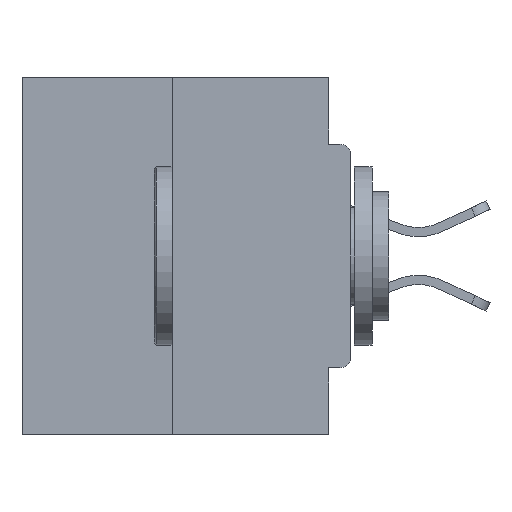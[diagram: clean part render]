
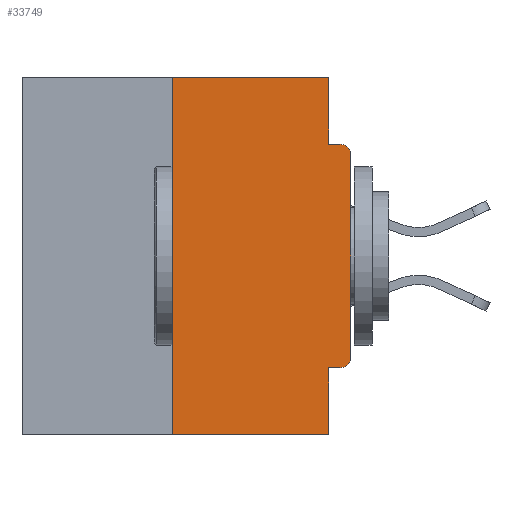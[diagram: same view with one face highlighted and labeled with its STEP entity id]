
A CAD part, left-side view. The second image highlights one B-rep face of the part: STEP entity #33749.
In plain terms, the highlighted planar face has unit normal (-1, 0, 0).
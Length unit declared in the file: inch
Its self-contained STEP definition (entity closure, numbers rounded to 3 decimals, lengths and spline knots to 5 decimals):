
#339 = DIRECTION ( 'NONE',  ( 0., 0., -1. ) ) ;
#529 = VERTEX_POINT ( 'NONE', #2302 ) ;
#733 = DIRECTION ( 'NONE',  ( 0., 0., -1. ) ) ;
#1420 = VECTOR ( 'NONE', #32001, 39.37008 ) ;
#1704 = CIRCLE ( 'NONE', #24526, 0.015 ) ;
#2302 = CARTESIAN_POINT ( 'NONE',  ( 0., 0.031, -0.5 ) ) ;
#2428 = VERTEX_POINT ( 'NONE', #33903 ) ;
#2849 = ORIENTED_EDGE ( 'NONE', *, *, #25005, .F. ) ;
#3294 = EDGE_CURVE ( 'NONE', #30026, #2428, #1704, .T. ) ;
#3412 = CARTESIAN_POINT ( 'NONE',  ( 0., 0.015, -0.3915 ) ) ;
#3542 = PLANE ( 'NONE',  #29094 ) ;
#4584 = ORIENTED_EDGE ( 'NONE', *, *, #19382, .F. ) ;
#4960 = CARTESIAN_POINT ( 'NONE',  ( 0., 0.46, 0. ) ) ;
#5961 = CARTESIAN_POINT ( 'NONE',  ( 0., 0., -0.0935 ) ) ;
#6824 = CARTESIAN_POINT ( 'NONE',  ( 0., 0.015, -0.1085 ) ) ;
#7089 = VECTOR ( 'NONE', #10782, 39.37008 ) ;
#8106 = LINE ( 'NONE', #30395, #28964 ) ;
#8495 = CARTESIAN_POINT ( 'NONE',  ( 0., 0.015, -0.4065 ) ) ;
#8805 = DIRECTION ( 'NONE',  ( 0., -1., 0. ) ) ;
#8964 = ORIENTED_EDGE ( 'NONE', *, *, #31930, .F. ) ;
#10055 = VECTOR ( 'NONE', #21540, 39.37008 ) ;
#10618 = CARTESIAN_POINT ( 'NONE',  ( 0., 0.25, 0. ) ) ;
#10782 = DIRECTION ( 'NONE',  ( 0., -1., 0. ) ) ;
#11637 = CIRCLE ( 'NONE', #35194, 0.015 ) ;
#11740 = ORIENTED_EDGE ( 'NONE', *, *, #20751, .T. ) ;
#13458 = VERTEX_POINT ( 'NONE', #14310 ) ;
#13988 = CARTESIAN_POINT ( 'NONE',  ( 0., 0.46, 0. ) ) ;
#14027 = DIRECTION ( 'NONE',  ( 0., 0., 1. ) ) ;
#14169 = DIRECTION ( 'NONE',  ( 0., 1., 0. ) ) ;
#14310 = CARTESIAN_POINT ( 'NONE',  ( 0., 0.031, -0.4065 ) ) ;
#15445 = CARTESIAN_POINT ( 'NONE',  ( 0., 0.015, -0.0935 ) ) ;
#15452 = CARTESIAN_POINT ( 'NONE',  ( 0., 0.031, 0. ) ) ;
#16321 = ORIENTED_EDGE ( 'NONE', *, *, #34888, .T. ) ;
#16607 = DIRECTION ( 'NONE',  ( 0., 0., -1. ) ) ;
#16608 = FACE_OUTER_BOUND ( 'NONE', #26049, .T. ) ;
#16656 = VECTOR ( 'NONE', #14169, 39.37008 ) ;
#17760 = EDGE_CURVE ( 'NONE', #19184, #34465, #28795, .T. ) ;
#18107 = DIRECTION ( 'NONE',  ( 0., 0., -1. ) ) ;
#18458 = EDGE_CURVE ( 'NONE', #34465, #23523, #22446, .T. ) ;
#18556 = LINE ( 'NONE', #5961, #33885 ) ;
#18764 = LINE ( 'NONE', #19774, #16656 ) ;
#19184 = VERTEX_POINT ( 'NONE', #27040 ) ;
#19209 = EDGE_CURVE ( 'NONE', #23523, #33570, #18556, .T. ) ;
#19382 = EDGE_CURVE ( 'NONE', #28916, #19184, #31724, .T. ) ;
#19695 = DIRECTION ( 'NONE',  ( -1., 0., 0. ) ) ;
#19774 = CARTESIAN_POINT ( 'NONE',  ( 0., 0., -0.4065 ) ) ;
#19952 = CARTESIAN_POINT ( 'NONE',  ( 0., 0.031, 0. ) ) ;
#20751 = EDGE_CURVE ( 'NONE', #25872, #33570, #11637, .T. ) ;
#21434 = CARTESIAN_POINT ( 'NONE',  ( 0., 0.25, -0.5 ) ) ;
#21540 = DIRECTION ( 'NONE',  ( 0., 0., 1. ) ) ;
#21894 = EDGE_CURVE ( 'NONE', #2428, #25872, #8106, .T. ) ;
#22035 = ORIENTED_EDGE ( 'NONE', *, *, #18458, .F. ) ;
#22446 = LINE ( 'NONE', #19952, #33483 ) ;
#23131 = DIRECTION ( 'NONE',  ( -1., 0., 0. ) ) ;
#23523 = VERTEX_POINT ( 'NONE', #34092 ) ;
#23684 = CARTESIAN_POINT ( 'NONE',  ( 0., 0.46, -0.5 ) ) ;
#23754 = CARTESIAN_POINT ( 'NONE',  ( 0., 0.031, -0.5 ) ) ;
#24526 = AXIS2_PLACEMENT_3D ( 'NONE', #3412, #19695, #16607 ) ;
#24997 = DIRECTION ( 'NONE',  ( 1., 0., 0. ) ) ;
#25005 = EDGE_CURVE ( 'NONE', #30026, #13458, #18764, .T. ) ;
#25858 = DIRECTION ( 'NONE',  ( 0., 0., -1. ) ) ;
#25872 = VERTEX_POINT ( 'NONE', #28402 ) ;
#26049 = EDGE_LOOP ( 'NONE', ( #27959, #4584, #16321, #8964, #2849, #28836, #30660, #11740, #32238, #22035 ) ) ;
#27040 = CARTESIAN_POINT ( 'NONE',  ( 0., 0.25, 0. ) ) ;
#27748 = LINE ( 'NONE', #23754, #27796 ) ;
#27796 = VECTOR ( 'NONE', #18107, 39.37008 ) ;
#27959 = ORIENTED_EDGE ( 'NONE', *, *, #17760, .F. ) ;
#28402 = CARTESIAN_POINT ( 'NONE',  ( 0., 0., -0.1085 ) ) ;
#28466 = LINE ( 'NONE', #23684, #1420 ) ;
#28795 = LINE ( 'NONE', #4960, #7089 ) ;
#28836 = ORIENTED_EDGE ( 'NONE', *, *, #3294, .T. ) ;
#28916 = VERTEX_POINT ( 'NONE', #21434 ) ;
#28964 = VECTOR ( 'NONE', #14027, 39.37008 ) ;
#29094 = AXIS2_PLACEMENT_3D ( 'NONE', #13988, #24997, #339 ) ;
#30026 = VERTEX_POINT ( 'NONE', #8495 ) ;
#30395 = CARTESIAN_POINT ( 'NONE',  ( 0., 0., 0. ) ) ;
#30660 = ORIENTED_EDGE ( 'NONE', *, *, #21894, .T. ) ;
#31724 = LINE ( 'NONE', #10618, #10055 ) ;
#31930 = EDGE_CURVE ( 'NONE', #13458, #529, #27748, .T. ) ;
#32001 = DIRECTION ( 'NONE',  ( 0., -1., 0. ) ) ;
#32238 = ORIENTED_EDGE ( 'NONE', *, *, #19209, .F. ) ;
#33483 = VECTOR ( 'NONE', #733, 39.37008 ) ;
#33570 = VERTEX_POINT ( 'NONE', #15445 ) ;
#33749 = ADVANCED_FACE ( 'NONE', ( #16608 ), #3542, .F. ) ;
#33885 = VECTOR ( 'NONE', #8805, 39.37008 ) ;
#33903 = CARTESIAN_POINT ( 'NONE',  ( 0., 0., -0.3915 ) ) ;
#34092 = CARTESIAN_POINT ( 'NONE',  ( 0., 0.031, -0.0935 ) ) ;
#34465 = VERTEX_POINT ( 'NONE', #15452 ) ;
#34888 = EDGE_CURVE ( 'NONE', #28916, #529, #28466, .T. ) ;
#35194 = AXIS2_PLACEMENT_3D ( 'NONE', #6824, #23131, #25858 ) ;
